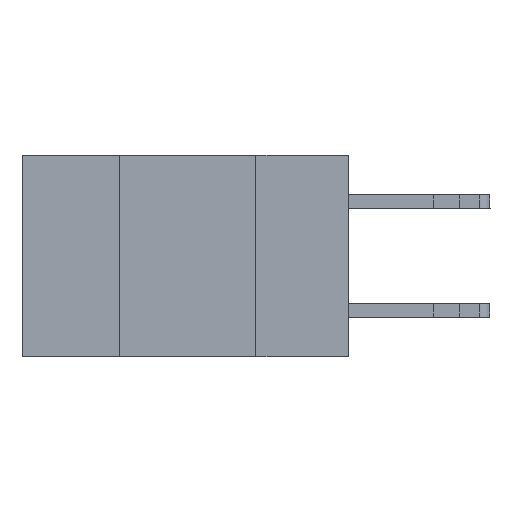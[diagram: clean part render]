
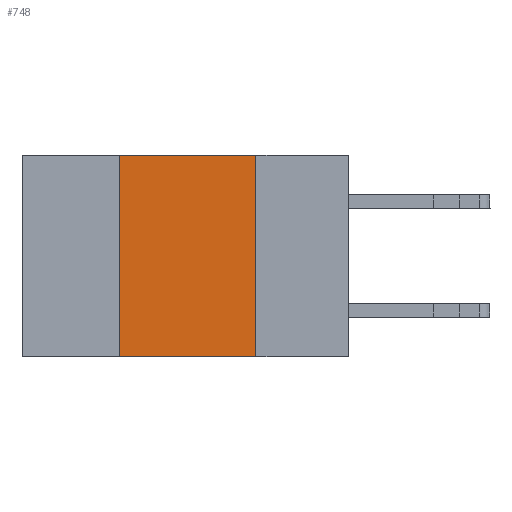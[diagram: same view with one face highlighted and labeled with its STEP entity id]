
A CAD part, left-side view. The second image highlights one B-rep face of the part: STEP entity #748.
In plain terms, the highlighted planar face has unit normal (-1, 0, 0).
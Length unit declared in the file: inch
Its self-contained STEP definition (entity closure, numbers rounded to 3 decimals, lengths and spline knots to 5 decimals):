
#748 = ADVANCED_FACE ( 'NONE', ( #6899 ), #3262, .F. ) ;
#756 = ORIENTED_EDGE ( 'NONE', *, *, #5453, .F. ) ;
#812 = CARTESIAN_POINT ( 'NONE',  ( 0., 0.42, -0.37 ) ) ;
#1273 = CARTESIAN_POINT ( 'NONE',  ( 0., 0.6, 0. ) ) ;
#1732 = ORIENTED_EDGE ( 'NONE', *, *, #13699, .T. ) ;
#1912 = AXIS2_PLACEMENT_3D ( 'NONE', #5668, #10587, #14313 ) ;
#3262 = PLANE ( 'NONE',  #1912 ) ;
#3633 = ORIENTED_EDGE ( 'NONE', *, *, #6599, .F. ) ;
#5453 = EDGE_CURVE ( 'NONE', #12982, #10357, #12434, .T. ) ;
#5528 = VECTOR ( 'NONE', #13559, 39.37008 ) ;
#5668 = CARTESIAN_POINT ( 'NONE',  ( 0., 0.6, 0. ) ) ;
#6129 = VECTOR ( 'NONE', #14117, 39.37008 ) ;
#6343 = VECTOR ( 'NONE', #6812, 39.37008 ) ;
#6599 = EDGE_CURVE ( 'NONE', #13424, #12982, #7050, .T. ) ;
#6812 = DIRECTION ( 'NONE',  ( 0., 0., 1. ) ) ;
#6899 = FACE_OUTER_BOUND ( 'NONE', #7558, .T. ) ;
#7050 = LINE ( 'NONE', #812, #6343 ) ;
#7558 = EDGE_LOOP ( 'NONE', ( #8397, #756, #3633, #1732 ) ) ;
#7826 = CARTESIAN_POINT ( 'NONE',  ( 0., 0.17, -0.37 ) ) ;
#8397 = ORIENTED_EDGE ( 'NONE', *, *, #11390, .F. ) ;
#9220 = LINE ( 'NONE', #9449, #15482 ) ;
#9245 = CARTESIAN_POINT ( 'NONE',  ( 0., 0.17, 0. ) ) ;
#9449 = CARTESIAN_POINT ( 'NONE',  ( 0., 0.6, -0.37 ) ) ;
#10357 = VERTEX_POINT ( 'NONE', #9245 ) ;
#10587 = DIRECTION ( 'NONE',  ( 1., 0., 0. ) ) ;
#11390 = EDGE_CURVE ( 'NONE', #10357, #14941, #11610, .T. ) ;
#11610 = LINE ( 'NONE', #7826, #6129 ) ;
#12434 = LINE ( 'NONE', #1273, #5528 ) ;
#12870 = DIRECTION ( 'NONE',  ( 0., -1., 0. ) ) ;
#12982 = VERTEX_POINT ( 'NONE', #13702 ) ;
#13424 = VERTEX_POINT ( 'NONE', #14793 ) ;
#13559 = DIRECTION ( 'NONE',  ( 0., -1., 0. ) ) ;
#13699 = EDGE_CURVE ( 'NONE', #13424, #14941, #9220, .T. ) ;
#13702 = CARTESIAN_POINT ( 'NONE',  ( 0., 0.42, 0. ) ) ;
#13926 = CARTESIAN_POINT ( 'NONE',  ( 0., 0.17, -0.37 ) ) ;
#14117 = DIRECTION ( 'NONE',  ( 0., 0., -1. ) ) ;
#14313 = DIRECTION ( 'NONE',  ( 0., 0., -1. ) ) ;
#14793 = CARTESIAN_POINT ( 'NONE',  ( 0., 0.42, -0.37 ) ) ;
#14941 = VERTEX_POINT ( 'NONE', #13926 ) ;
#15482 = VECTOR ( 'NONE', #12870, 39.37008 ) ;
